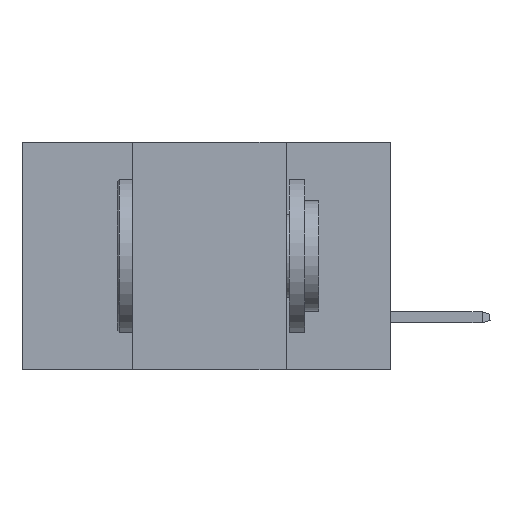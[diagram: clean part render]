
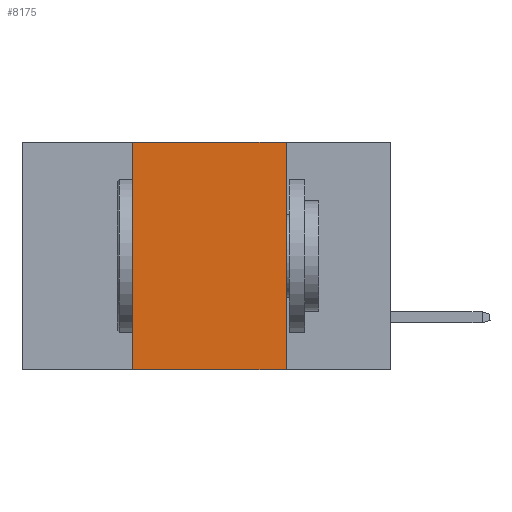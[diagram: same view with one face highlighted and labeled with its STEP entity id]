
A CAD part, left-side view. The second image highlights one B-rep face of the part: STEP entity #8175.
In plain terms, the highlighted planar face has unit normal (-1, 0, 0).
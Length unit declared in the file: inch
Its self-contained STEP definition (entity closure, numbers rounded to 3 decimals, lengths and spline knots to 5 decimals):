
#3534 = ORIENTED_EDGE ( 'NONE', *, *, #41659, .F. ) ;
#3596 = CARTESIAN_POINT ( 'NONE',  ( 0., 0.42, -0.37 ) ) ;
#3688 = DIRECTION ( 'NONE',  ( 0., 0., -1. ) ) ;
#5475 = ORIENTED_EDGE ( 'NONE', *, *, #17477, .T. ) ;
#5906 = CARTESIAN_POINT ( 'NONE',  ( 0., 0.42, 0. ) ) ;
#8175 = ADVANCED_FACE ( 'NONE', ( #26454 ), #18825, .F. ) ;
#8269 = DIRECTION ( 'NONE',  ( 1., 0., 0. ) ) ;
#8312 = VERTEX_POINT ( 'NONE', #29546 ) ;
#9336 = ORIENTED_EDGE ( 'NONE', *, *, #15711, .F. ) ;
#12208 = AXIS2_PLACEMENT_3D ( 'NONE', #43385, #8269, #14836 ) ;
#14836 = DIRECTION ( 'NONE',  ( 0., 0., -1. ) ) ;
#15711 = EDGE_CURVE ( 'NONE', #17109, #16382, #22183, .T. ) ;
#16382 = VERTEX_POINT ( 'NONE', #27829 ) ;
#17109 = VERTEX_POINT ( 'NONE', #43675 ) ;
#17477 = EDGE_CURVE ( 'NONE', #36869, #16382, #33576, .T. ) ;
#18224 = EDGE_CURVE ( 'NONE', #8312, #17109, #31271, .T. ) ;
#18825 = PLANE ( 'NONE',  #12208 ) ;
#20814 = CARTESIAN_POINT ( 'NONE',  ( 0., 0.17, 0. ) ) ;
#21896 = EDGE_LOOP ( 'NONE', ( #9336, #22271, #3534, #5475 ) ) ;
#22183 = LINE ( 'NONE', #20814, #28790 ) ;
#22271 = ORIENTED_EDGE ( 'NONE', *, *, #18224, .F. ) ;
#24282 = DIRECTION ( 'NONE',  ( 0., -1., 0. ) ) ;
#25037 = VECTOR ( 'NONE', #27026, 39.37008 ) ;
#26454 = FACE_OUTER_BOUND ( 'NONE', #21896, .T. ) ;
#26989 = VECTOR ( 'NONE', #24282, 39.37008 ) ;
#27026 = DIRECTION ( 'NONE',  ( 0., 0., 1. ) ) ;
#27829 = CARTESIAN_POINT ( 'NONE',  ( 0., 0.17, -0.37 ) ) ;
#28790 = VECTOR ( 'NONE', #3688, 39.37008 ) ;
#29148 = DIRECTION ( 'NONE',  ( 0., -1., 0. ) ) ;
#29546 = CARTESIAN_POINT ( 'NONE',  ( 0., 0.42, 0. ) ) ;
#31271 = LINE ( 'NONE', #32500, #42282 ) ;
#32500 = CARTESIAN_POINT ( 'NONE',  ( 0., 0.6, 0. ) ) ;
#33576 = LINE ( 'NONE', #34673, #26989 ) ;
#34673 = CARTESIAN_POINT ( 'NONE',  ( 0., 0.6, -0.37 ) ) ;
#36869 = VERTEX_POINT ( 'NONE', #3596 ) ;
#38173 = LINE ( 'NONE', #5906, #25037 ) ;
#41659 = EDGE_CURVE ( 'NONE', #36869, #8312, #38173, .T. ) ;
#42282 = VECTOR ( 'NONE', #29148, 39.37008 ) ;
#43385 = CARTESIAN_POINT ( 'NONE',  ( 0., 0.6, 0. ) ) ;
#43675 = CARTESIAN_POINT ( 'NONE',  ( 0., 0.17, 0. ) ) ;
